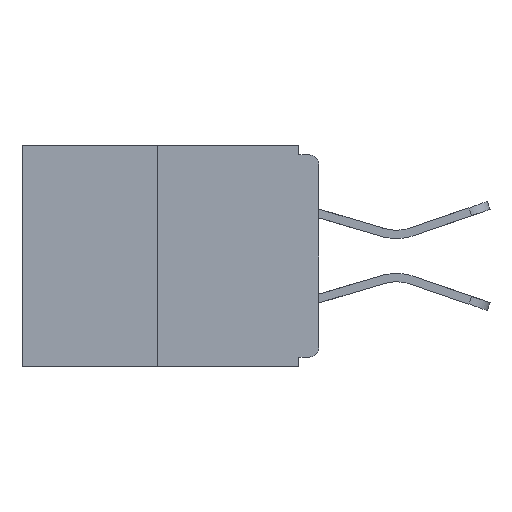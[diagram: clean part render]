
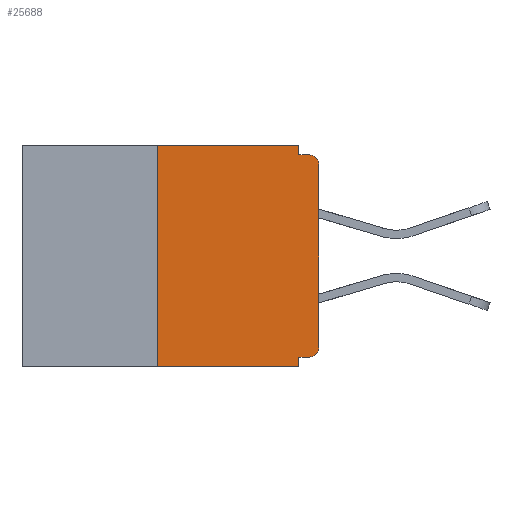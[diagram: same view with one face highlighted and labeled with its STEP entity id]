
A CAD part, left-side view. The second image highlights one B-rep face of the part: STEP entity #25688.
In plain terms, the highlighted planar face has unit normal (-1, 0, 0).
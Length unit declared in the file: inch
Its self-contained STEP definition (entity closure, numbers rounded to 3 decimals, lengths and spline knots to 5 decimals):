
#244 = LINE ( 'NONE', #21184, #21071 ) ;
#495 = LINE ( 'NONE', #22470, #4924 ) ;
#591 = DIRECTION ( 'NONE',  ( 0., 0., -1. ) ) ;
#1235 = VECTOR ( 'NONE', #16634, 39.37008 ) ;
#3095 = CARTESIAN_POINT ( 'NONE',  ( 0., 0.031, -0.015 ) ) ;
#3405 = LINE ( 'NONE', #7630, #19181 ) ;
#3577 = CARTESIAN_POINT ( 'NONE',  ( 0., 0.25, -0.343 ) ) ;
#3936 = ORIENTED_EDGE ( 'NONE', *, *, #12403, .T. ) ;
#4924 = VECTOR ( 'NONE', #19841, 39.37008 ) ;
#5187 = ORIENTED_EDGE ( 'NONE', *, *, #25029, .T. ) ;
#5593 = EDGE_CURVE ( 'NONE', #8773, #15816, #6259, .T. ) ;
#5755 = EDGE_CURVE ( 'NONE', #19866, #22687, #244, .T. ) ;
#6079 = CARTESIAN_POINT ( 'NONE',  ( 0., 0.015, -0.03 ) ) ;
#6218 = CIRCLE ( 'NONE', #19786, 0.015 ) ;
#6259 = LINE ( 'NONE', #20400, #22053 ) ;
#6451 = VERTEX_POINT ( 'NONE', #7258 ) ;
#6470 = VECTOR ( 'NONE', #19016, 39.37008 ) ;
#6556 = DIRECTION ( 'NONE',  ( 0., -1., 0. ) ) ;
#7258 = CARTESIAN_POINT ( 'NONE',  ( 0., 0.031, -0.343 ) ) ;
#7570 = VERTEX_POINT ( 'NONE', #19105 ) ;
#7630 = CARTESIAN_POINT ( 'NONE',  ( 0., 0.46, -0.343 ) ) ;
#7901 = LINE ( 'NONE', #18406, #1235 ) ;
#8283 = CARTESIAN_POINT ( 'NONE',  ( 0., 0., -0.03 ) ) ;
#8653 = CARTESIAN_POINT ( 'NONE',  ( 0., 0.015, -0.313 ) ) ;
#8773 = VERTEX_POINT ( 'NONE', #3095 ) ;
#8792 = PLANE ( 'NONE',  #9232 ) ;
#9232 = AXIS2_PLACEMENT_3D ( 'NONE', #16835, #16652, #18674 ) ;
#9785 = ORIENTED_EDGE ( 'NONE', *, *, #22798, .T. ) ;
#10366 = VERTEX_POINT ( 'NONE', #23146 ) ;
#10680 = DIRECTION ( 'NONE',  ( -1., 0., 0. ) ) ;
#10812 = VERTEX_POINT ( 'NONE', #18798 ) ;
#10985 = ORIENTED_EDGE ( 'NONE', *, *, #17163, .F. ) ;
#11015 = ORIENTED_EDGE ( 'NONE', *, *, #13081, .T. ) ;
#11202 = ORIENTED_EDGE ( 'NONE', *, *, #14086, .F. ) ;
#11600 = ORIENTED_EDGE ( 'NONE', *, *, #5593, .F. ) ;
#11691 = DIRECTION ( 'NONE',  ( 0., 0., -1. ) ) ;
#12403 = EDGE_CURVE ( 'NONE', #10366, #21570, #7901, .T. ) ;
#12845 = ORIENTED_EDGE ( 'NONE', *, *, #5755, .F. ) ;
#13081 = EDGE_CURVE ( 'NONE', #19866, #6451, #3405, .T. ) ;
#13299 = VERTEX_POINT ( 'NONE', #16620 ) ;
#13569 = DIRECTION ( 'NONE',  ( 0., -1., 0. ) ) ;
#13574 = ORIENTED_EDGE ( 'NONE', *, *, #21251, .F. ) ;
#13856 = LINE ( 'NONE', #16971, #25436 ) ;
#14086 = EDGE_CURVE ( 'NONE', #7570, #6451, #495, .T. ) ;
#14408 = EDGE_LOOP ( 'NONE', ( #14705, #12845, #11015, #11202, #13574, #5187, #3936, #9785, #11600, #10985 ) ) ;
#14705 = ORIENTED_EDGE ( 'NONE', *, *, #22953, .F. ) ;
#14977 = LINE ( 'NONE', #23906, #24098 ) ;
#15816 = VERTEX_POINT ( 'NONE', #19275 ) ;
#16323 = DIRECTION ( 'NONE',  ( -1., 0., 0. ) ) ;
#16620 = CARTESIAN_POINT ( 'NONE',  ( 0., 0.031, 0. ) ) ;
#16634 = DIRECTION ( 'NONE',  ( 0., 0., 1. ) ) ;
#16652 = DIRECTION ( 'NONE',  ( 1., 0., 0. ) ) ;
#16835 = CARTESIAN_POINT ( 'NONE',  ( 0., 0.46, 0. ) ) ;
#16971 = CARTESIAN_POINT ( 'NONE',  ( 0., 0., -0.328 ) ) ;
#17141 = DIRECTION ( 'NONE',  ( 0., 1., 0. ) ) ;
#17163 = EDGE_CURVE ( 'NONE', #13299, #8773, #14977, .T. ) ;
#18406 = CARTESIAN_POINT ( 'NONE',  ( 0., 0., 0. ) ) ;
#18674 = DIRECTION ( 'NONE',  ( 0., 0., -1. ) ) ;
#18798 = CARTESIAN_POINT ( 'NONE',  ( 0., 0.015, -0.328 ) ) ;
#18988 = CIRCLE ( 'NONE', #19321, 0.015 ) ;
#19016 = DIRECTION ( 'NONE',  ( 0., -1., 0. ) ) ;
#19105 = CARTESIAN_POINT ( 'NONE',  ( 0., 0.031, -0.328 ) ) ;
#19181 = VECTOR ( 'NONE', #13569, 39.37008 ) ;
#19275 = CARTESIAN_POINT ( 'NONE',  ( 0., 0.015, -0.015 ) ) ;
#19321 = AXIS2_PLACEMENT_3D ( 'NONE', #8653, #10680, #591 ) ;
#19786 = AXIS2_PLACEMENT_3D ( 'NONE', #6079, #16323, #24384 ) ;
#19841 = DIRECTION ( 'NONE',  ( 0., 0., -1. ) ) ;
#19866 = VERTEX_POINT ( 'NONE', #3577 ) ;
#20400 = CARTESIAN_POINT ( 'NONE',  ( 0., 0., -0.015 ) ) ;
#21071 = VECTOR ( 'NONE', #25063, 39.37008 ) ;
#21184 = CARTESIAN_POINT ( 'NONE',  ( 0., 0.25, 0. ) ) ;
#21251 = EDGE_CURVE ( 'NONE', #10812, #7570, #13856, .T. ) ;
#21287 = CARTESIAN_POINT ( 'NONE',  ( 0., 0.46, 0. ) ) ;
#21570 = VERTEX_POINT ( 'NONE', #8283 ) ;
#22053 = VECTOR ( 'NONE', #6556, 39.37008 ) ;
#22470 = CARTESIAN_POINT ( 'NONE',  ( 0., 0.031, -0.343 ) ) ;
#22687 = VERTEX_POINT ( 'NONE', #24466 ) ;
#22798 = EDGE_CURVE ( 'NONE', #21570, #15816, #6218, .T. ) ;
#22953 = EDGE_CURVE ( 'NONE', #22687, #13299, #23509, .T. ) ;
#23146 = CARTESIAN_POINT ( 'NONE',  ( 0., 0., -0.313 ) ) ;
#23509 = LINE ( 'NONE', #21287, #6470 ) ;
#23906 = CARTESIAN_POINT ( 'NONE',  ( 0., 0.031, 0. ) ) ;
#23995 = FACE_OUTER_BOUND ( 'NONE', #14408, .T. ) ;
#24098 = VECTOR ( 'NONE', #11691, 39.37008 ) ;
#24384 = DIRECTION ( 'NONE',  ( 0., 0., -1. ) ) ;
#24466 = CARTESIAN_POINT ( 'NONE',  ( 0., 0.25, 0. ) ) ;
#25029 = EDGE_CURVE ( 'NONE', #10812, #10366, #18988, .T. ) ;
#25063 = DIRECTION ( 'NONE',  ( 0., 0., 1. ) ) ;
#25436 = VECTOR ( 'NONE', #17141, 39.37008 ) ;
#25688 = ADVANCED_FACE ( 'NONE', ( #23995 ), #8792, .F. ) ;
